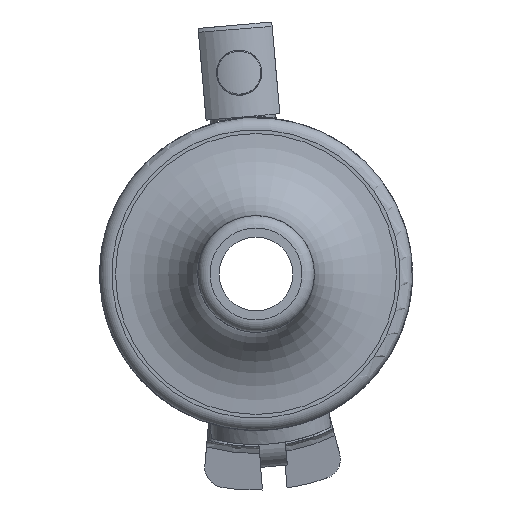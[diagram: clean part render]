
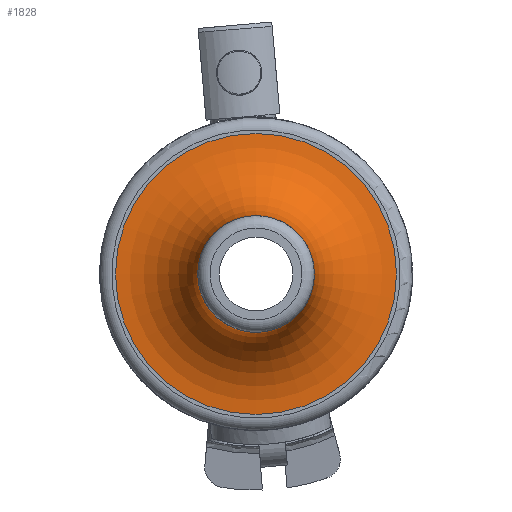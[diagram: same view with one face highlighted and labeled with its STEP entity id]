
A CAD part, left-side view. The second image highlights one B-rep face of the part: STEP entity #1828.
In plain terms, the highlighted toroidal (fillet/blend) face has major radius 17.1 mm and minor radius 10 mm.
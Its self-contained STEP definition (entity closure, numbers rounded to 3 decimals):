
#22=TOROIDAL_SURFACE('',#1967,17.1,10.);
#233=FACE_OUTER_BOUND('',#346,.T.);
#346=EDGE_LOOP('',(#1409,#1410,#1411,#1412,#1413));
#700=CIRCLE('',#1968,17.1);
#701=CIRCLE('',#1969,10.);
#702=CIRCLE('',#1970,7.1);
#703=CIRCLE('',#1971,7.1);
#820=VERTEX_POINT('',#3914);
#821=VERTEX_POINT('',#3916);
#822=VERTEX_POINT('',#3918);
#1035=EDGE_CURVE('',#820,#820,#700,.T.);
#1036=EDGE_CURVE('',#820,#821,#701,.T.);
#1037=EDGE_CURVE('',#821,#822,#702,.T.);
#1038=EDGE_CURVE('',#822,#821,#703,.T.);
#1409=ORIENTED_EDGE('',*,*,#1035,.T.);
#1410=ORIENTED_EDGE('',*,*,#1036,.T.);
#1411=ORIENTED_EDGE('',*,*,#1037,.T.);
#1412=ORIENTED_EDGE('',*,*,#1038,.T.);
#1413=ORIENTED_EDGE('',*,*,#1036,.F.);
#1828=ADVANCED_FACE('',(#233),#22,.F.);
#1967=AXIS2_PLACEMENT_3D('',#3913,#2249,#2250);
#1968=AXIS2_PLACEMENT_3D('',#3915,#2251,#2252);
#1969=AXIS2_PLACEMENT_3D('',#3917,#2253,#2254);
#1970=AXIS2_PLACEMENT_3D('',#3919,#2255,#2256);
#1971=AXIS2_PLACEMENT_3D('',#3920,#2257,#2258);
#2249=DIRECTION('center_axis',(1.,0.,0.));
#2250=DIRECTION('ref_axis',(0.,0.,-1.));
#2251=DIRECTION('center_axis',(-1.,0.,0.));
#2252=DIRECTION('ref_axis',(0.,-0.94,0.342));
#2253=DIRECTION('center_axis',(0.,1.,0.));
#2254=DIRECTION('ref_axis',(0.,0.,1.));
#2255=DIRECTION('center_axis',(1.,0.,0.));
#2256=DIRECTION('ref_axis',(0.,-0.94,0.342));
#2257=DIRECTION('center_axis',(1.,0.,0.));
#2258=DIRECTION('ref_axis',(0.,-0.94,0.342));
#3913=CARTESIAN_POINT('Origin',(-94.5,26.227,197.771));
#3914=CARTESIAN_POINT('',(-84.5,26.227,214.871));
#3915=CARTESIAN_POINT('Origin',(-84.5,26.227,197.771));
#3916=CARTESIAN_POINT('',(-94.5,26.227,204.871));
#3917=CARTESIAN_POINT('Origin',(-94.5,26.227,214.871));
#3918=CARTESIAN_POINT('',(-94.5,32.898,195.343));
#3919=CARTESIAN_POINT('Origin',(-94.5,26.227,197.771));
#3920=CARTESIAN_POINT('Origin',(-94.5,26.227,197.771));
